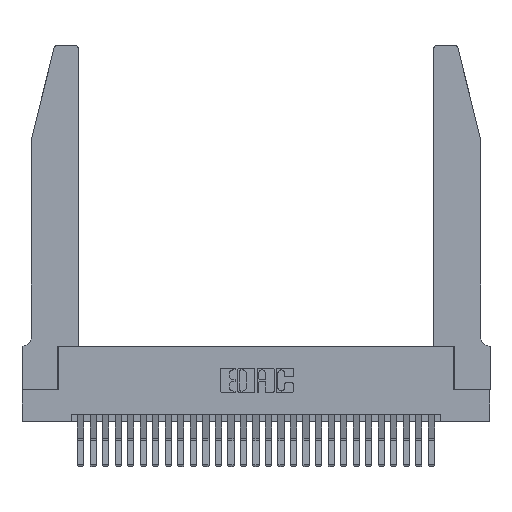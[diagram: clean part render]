
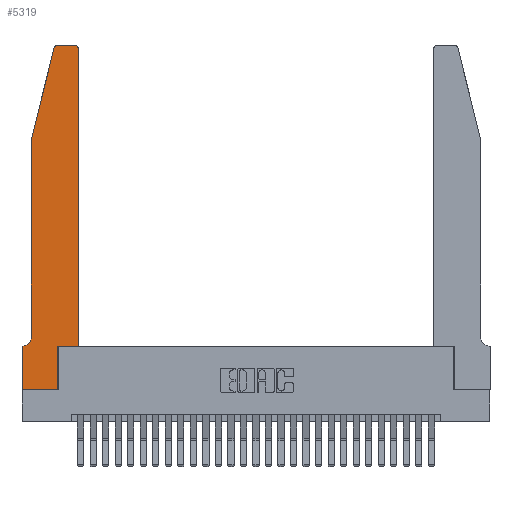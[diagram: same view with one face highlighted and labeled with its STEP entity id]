
A CAD part, top view. The second image highlights one B-rep face of the part: STEP entity #5319.
In plain terms, the highlighted planar face has unit normal (0, 0, 1).
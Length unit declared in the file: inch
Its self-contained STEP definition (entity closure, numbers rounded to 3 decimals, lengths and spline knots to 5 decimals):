
#252 = FACE_OUTER_BOUND ( 'NONE', #13085, .T. ) ;
#286 = CARTESIAN_POINT ( 'NONE',  ( 0.4505, 0.35, 0.37 ) ) ;
#1104 = VECTOR ( 'NONE', #17027, 39.37008 ) ;
#1591 = AXIS2_PLACEMENT_3D ( 'NONE', #2442, #18602, #4809 ) ;
#1826 = LINE ( 'NONE', #3682, #25339 ) ;
#2186 = VECTOR ( 'NONE', #10828, 39.37008 ) ;
#2377 = EDGE_CURVE ( 'NONE', #19143, #26219, #19405, .T. ) ;
#2442 = CARTESIAN_POINT ( 'NONE',  ( 0.4205, 2.72, 0.37 ) ) ;
#2631 = DIRECTION ( 'NONE',  ( 0., 1., 0. ) ) ;
#2671 = VERTEX_POINT ( 'NONE', #3624 ) ;
#3226 = EDGE_CURVE ( 'NONE', #5255, #11896, #24528, .T. ) ;
#3336 = ORIENTED_EDGE ( 'NONE', *, *, #5365, .T. ) ;
#3624 = CARTESIAN_POINT ( 'NONE',  ( 0.4205, 2.75, 0.37 ) ) ;
#3682 = CARTESIAN_POINT ( 'NONE',  ( 0.2865, 0.35, 0.37 ) ) ;
#4601 = CARTESIAN_POINT ( 'NONE',  ( 0.0755, 2., 0.37 ) ) ;
#4809 = DIRECTION ( 'NONE',  ( 1., 0., 0. ) ) ;
#4826 = ORIENTED_EDGE ( 'NONE', *, *, #2377, .T. ) ;
#4942 = CARTESIAN_POINT ( 'NONE',  ( 0.0755, 0.35, 0.37 ) ) ;
#5037 = VECTOR ( 'NONE', #28728, 39.37008 ) ;
#5255 = VERTEX_POINT ( 'NONE', #7611 ) ;
#5319 = ADVANCED_FACE ( 'NONE', ( #252 ), #19279, .T. ) ;
#5365 = EDGE_CURVE ( 'NONE', #10748, #20243, #16548, .T. ) ;
#5423 = CARTESIAN_POINT ( 'NONE',  ( 0.4505, 0.35, 0.37 ) ) ;
#5509 = DIRECTION ( 'NONE',  ( 0., 0., 1. ) ) ;
#5557 = CARTESIAN_POINT ( 'NONE',  ( 0.0755, 2., 0.37 ) ) ;
#6332 = CARTESIAN_POINT ( 'NONE',  ( 0.284, 2.72, 0.37 ) ) ;
#6460 = EDGE_CURVE ( 'NONE', #15956, #14021, #20363, .T. ) ;
#6604 = ORIENTED_EDGE ( 'NONE', *, *, #28456, .T. ) ;
#7611 = CARTESIAN_POINT ( 'NONE',  ( 0.2865, 0.35, 0.37 ) ) ;
#7833 = VECTOR ( 'NONE', #21386, 39.37008 ) ;
#7916 = VERTEX_POINT ( 'NONE', #18843 ) ;
#7922 = VECTOR ( 'NONE', #9414, 39.37008 ) ;
#8430 = ORIENTED_EDGE ( 'NONE', *, *, #28565, .T. ) ;
#8562 = VECTOR ( 'NONE', #23165, 39.37008 ) ;
#8655 = DIRECTION ( 'NONE',  ( 1., 0., 0. ) ) ;
#9075 = EDGE_CURVE ( 'NONE', #7916, #2671, #10217, .T. ) ;
#9343 = CARTESIAN_POINT ( 'NONE',  ( 0., 0.35, 0.37 ) ) ;
#9414 = DIRECTION ( 'NONE',  ( -1., 0., 0. ) ) ;
#9514 = ORIENTED_EDGE ( 'NONE', *, *, #20303, .T. ) ;
#9977 = LINE ( 'NONE', #286, #16124 ) ;
#10217 = CIRCLE ( 'NONE', #1591, 0.03 ) ;
#10561 = EDGE_CURVE ( 'NONE', #26219, #5255, #1826, .T. ) ;
#10748 = VERTEX_POINT ( 'NONE', #22572 ) ;
#10828 = DIRECTION ( 'NONE',  ( 0., -1., 0. ) ) ;
#10903 = ORIENTED_EDGE ( 'NONE', *, *, #10561, .T. ) ;
#11249 = ORIENTED_EDGE ( 'NONE', *, *, #6460, .T. ) ;
#11482 = EDGE_CURVE ( 'NONE', #2671, #15956, #20797, .T. ) ;
#11896 = VERTEX_POINT ( 'NONE', #26268 ) ;
#12058 = VERTEX_POINT ( 'NONE', #24646 ) ;
#12607 = CARTESIAN_POINT ( 'NONE',  ( 0.0055, 0.42, 0.37 ) ) ;
#13085 = EDGE_LOOP ( 'NONE', ( #28449, #11249, #6604, #26072, #3336, #9514, #16355, #4826, #10903, #18523, #8430, #14539 ) ) ;
#13286 = CARTESIAN_POINT ( 'NONE',  ( 0.25487, 2.72718, 0.37 ) ) ;
#13940 = LINE ( 'NONE', #4942, #8562 ) ;
#14021 = VERTEX_POINT ( 'NONE', #13286 ) ;
#14539 = ORIENTED_EDGE ( 'NONE', *, *, #9075, .T. ) ;
#14679 = AXIS2_PLACEMENT_3D ( 'NONE', #25806, #5509, #21466 ) ;
#14898 = CARTESIAN_POINT ( 'NONE',  ( 0., 0., 0.37 ) ) ;
#14948 = DIRECTION ( 'NONE',  ( -1., 0., 0. ) ) ;
#15956 = VERTEX_POINT ( 'NONE', #19045 ) ;
#16124 = VECTOR ( 'NONE', #2631, 39.37008 ) ;
#16223 = CARTESIAN_POINT ( 'NONE',  ( 0.0055, 0.35, 0.37 ) ) ;
#16355 = ORIENTED_EDGE ( 'NONE', *, *, #23261, .T. ) ;
#16548 = CIRCLE ( 'NONE', #20765, 0.07 ) ;
#17027 = DIRECTION ( 'NONE',  ( 0., -1., 0. ) ) ;
#17566 = VECTOR ( 'NONE', #27228, 39.37008 ) ;
#17611 = AXIS2_PLACEMENT_3D ( 'NONE', #6332, #22293, #8655 ) ;
#18523 = ORIENTED_EDGE ( 'NONE', *, *, #3226, .T. ) ;
#18602 = DIRECTION ( 'NONE',  ( 0., 0., 1. ) ) ;
#18843 = CARTESIAN_POINT ( 'NONE',  ( 0.4505, 2.72, 0.37 ) ) ;
#19045 = CARTESIAN_POINT ( 'NONE',  ( 0.284, 2.75, 0.37 ) ) ;
#19136 = LINE ( 'NONE', #22194, #2186 ) ;
#19143 = VERTEX_POINT ( 'NONE', #20611 ) ;
#19279 = PLANE ( 'NONE',  #14679 ) ;
#19405 = LINE ( 'NONE', #14898, #5037 ) ;
#19774 = DIRECTION ( 'NONE',  ( 0., 1., 0. ) ) ;
#20243 = VERTEX_POINT ( 'NONE', #16223 ) ;
#20303 = EDGE_CURVE ( 'NONE', #20243, #28520, #13940, .T. ) ;
#20363 = CIRCLE ( 'NONE', #17611, 0.03 ) ;
#20611 = CARTESIAN_POINT ( 'NONE',  ( 0., 0., 0.37 ) ) ;
#20765 = AXIS2_PLACEMENT_3D ( 'NONE', #12607, #28270, #14948 ) ;
#20797 = LINE ( 'NONE', #27393, #7922 ) ;
#21386 = DIRECTION ( 'NONE',  ( 1., 0., 0. ) ) ;
#21466 = DIRECTION ( 'NONE',  ( 1., 0., 0. ) ) ;
#22194 = CARTESIAN_POINT ( 'NONE',  ( 0., 0., 0.37 ) ) ;
#22293 = DIRECTION ( 'NONE',  ( 0., 0., 1. ) ) ;
#22572 = CARTESIAN_POINT ( 'NONE',  ( 0.0755, 0.42, 0.37 ) ) ;
#23074 = EDGE_CURVE ( 'NONE', #12058, #10748, #25355, .T. ) ;
#23165 = DIRECTION ( 'NONE',  ( -1., 0., 0. ) ) ;
#23261 = EDGE_CURVE ( 'NONE', #28520, #19143, #19136, .T. ) ;
#23470 = LINE ( 'NONE', #4601, #17566 ) ;
#23770 = CARTESIAN_POINT ( 'NONE',  ( 0.2865, 0., 0.37 ) ) ;
#24528 = LINE ( 'NONE', #5423, #7833 ) ;
#24646 = CARTESIAN_POINT ( 'NONE',  ( 0.0755, 2., 0.37 ) ) ;
#25339 = VECTOR ( 'NONE', #19774, 39.37008 ) ;
#25355 = LINE ( 'NONE', #5557, #1104 ) ;
#25806 = CARTESIAN_POINT ( 'NONE',  ( 0., 0.35, 0.37 ) ) ;
#26072 = ORIENTED_EDGE ( 'NONE', *, *, #23074, .T. ) ;
#26219 = VERTEX_POINT ( 'NONE', #23770 ) ;
#26268 = CARTESIAN_POINT ( 'NONE',  ( 0.4505, 0.35, 0.37 ) ) ;
#27228 = DIRECTION ( 'NONE',  ( -0.239, -0.971, 0. ) ) ;
#27393 = CARTESIAN_POINT ( 'NONE',  ( 0.2605, 2.75, 0.37 ) ) ;
#28270 = DIRECTION ( 'NONE',  ( 0., 0., -1. ) ) ;
#28449 = ORIENTED_EDGE ( 'NONE', *, *, #11482, .T. ) ;
#28456 = EDGE_CURVE ( 'NONE', #14021, #12058, #23470, .T. ) ;
#28520 = VERTEX_POINT ( 'NONE', #9343 ) ;
#28565 = EDGE_CURVE ( 'NONE', #11896, #7916, #9977, .T. ) ;
#28728 = DIRECTION ( 'NONE',  ( 1., 0., 0. ) ) ;
